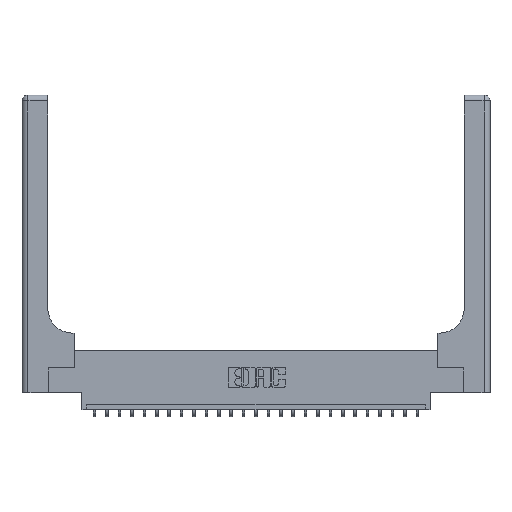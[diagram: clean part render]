
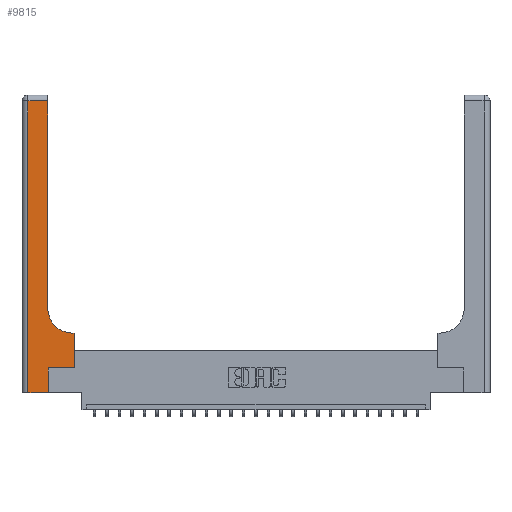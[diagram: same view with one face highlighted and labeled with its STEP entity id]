
A CAD part, top view. The second image highlights one B-rep face of the part: STEP entity #9815.
In plain terms, the highlighted planar face has unit normal (0, 0, 1).
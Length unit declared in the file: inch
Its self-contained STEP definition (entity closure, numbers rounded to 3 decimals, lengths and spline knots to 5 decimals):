
#491 = ORIENTED_EDGE ( 'NONE', *, *, #1760, .T. ) ;
#774 = PLANE ( 'NONE',  #8479 ) ;
#1011 = CIRCLE ( 'NONE', #23715, 0.25 ) ;
#1182 = LINE ( 'NONE', #22111, #23759 ) ;
#1273 = ORIENTED_EDGE ( 'NONE', *, *, #3967, .T. ) ;
#1760 = EDGE_CURVE ( 'NONE', #19154, #17649, #5342, .T. ) ;
#2073 = LINE ( 'NONE', #9685, #15956 ) ;
#2441 = DIRECTION ( 'NONE',  ( 1., 0., 0. ) ) ;
#2505 = CARTESIAN_POINT ( 'NONE',  ( 0.51, 0.85, 0.37 ) ) ;
#2872 = VERTEX_POINT ( 'NONE', #9540 ) ;
#3094 = EDGE_LOOP ( 'NONE', ( #10703, #1273, #18978, #21468, #18209, #21316, #21312, #491, #20974 ) ) ;
#3801 = CARTESIAN_POINT ( 'NONE',  ( 0.06, 2.94, 0.37 ) ) ;
#3824 = VERTEX_POINT ( 'NONE', #4258 ) ;
#3967 = EDGE_CURVE ( 'NONE', #21462, #16790, #12700, .T. ) ;
#4244 = CARTESIAN_POINT ( 'NONE',  ( 0.06, 0., 0.37 ) ) ;
#4258 = CARTESIAN_POINT ( 'NONE',  ( 0.26, 0.85, 0.37 ) ) ;
#5223 = CARTESIAN_POINT ( 'NONE',  ( 0.528, 0.25, 0.37 ) ) ;
#5342 = LINE ( 'NONE', #15129, #18626 ) ;
#5750 = VERTEX_POINT ( 'NONE', #5223 ) ;
#6818 = DIRECTION ( 'NONE',  ( 0., 1., 0. ) ) ;
#6942 = LINE ( 'NONE', #23510, #23726 ) ;
#8479 = AXIS2_PLACEMENT_3D ( 'NONE', #19824, #8750, #10242 ) ;
#8647 = EDGE_CURVE ( 'NONE', #17649, #3824, #1011, .T. ) ;
#8750 = DIRECTION ( 'NONE',  ( 0., 0., -1. ) ) ;
#9474 = CARTESIAN_POINT ( 'NONE',  ( 0.26, 2.94, 0.37 ) ) ;
#9540 = CARTESIAN_POINT ( 'NONE',  ( 0.265, 0., 0.37 ) ) ;
#9685 = CARTESIAN_POINT ( 'NONE',  ( 0., 0., 0.37 ) ) ;
#9815 = ADVANCED_FACE ( 'NONE', ( #21569 ), #774, .F. ) ;
#9930 = CARTESIAN_POINT ( 'NONE',  ( 0.528, 0.6, 0.37 ) ) ;
#10104 = VECTOR ( 'NONE', #24048, 39.37008 ) ;
#10111 = DIRECTION ( 'NONE',  ( 1., 0., 0. ) ) ;
#10190 = VECTOR ( 'NONE', #23112, 39.37008 ) ;
#10242 = DIRECTION ( 'NONE',  ( -1., 0., 0. ) ) ;
#10245 = VERTEX_POINT ( 'NONE', #17662 ) ;
#10475 = CARTESIAN_POINT ( 'NONE',  ( 0., 2.94, 0.37 ) ) ;
#10532 = DIRECTION ( 'NONE',  ( 1., 0., 0. ) ) ;
#10703 = ORIENTED_EDGE ( 'NONE', *, *, #14187, .T. ) ;
#11820 = LINE ( 'NONE', #21167, #16382 ) ;
#12235 = CARTESIAN_POINT ( 'NONE',  ( 0.51, 0.6, 0.37 ) ) ;
#12700 = LINE ( 'NONE', #10475, #10104 ) ;
#14187 = EDGE_CURVE ( 'NONE', #3824, #21462, #6942, .T. ) ;
#14262 = LINE ( 'NONE', #14742, #19322 ) ;
#14393 = EDGE_CURVE ( 'NONE', #5750, #19154, #22991, .T. ) ;
#14742 = CARTESIAN_POINT ( 'NONE',  ( 0.06, 3., 0.37 ) ) ;
#15129 = CARTESIAN_POINT ( 'NONE',  ( 0.26, 0.6, 0.37 ) ) ;
#15630 = EDGE_CURVE ( 'NONE', #16790, #20341, #14262, .T. ) ;
#15956 = VECTOR ( 'NONE', #2441, 39.37008 ) ;
#16382 = VECTOR ( 'NONE', #19300, 39.37008 ) ;
#16790 = VERTEX_POINT ( 'NONE', #3801 ) ;
#16891 = DIRECTION ( 'NONE',  ( -1., 0., 0. ) ) ;
#17111 = CARTESIAN_POINT ( 'NONE',  ( 0.528, 0.25, 0.37 ) ) ;
#17148 = EDGE_CURVE ( 'NONE', #10245, #5750, #1182, .T. ) ;
#17649 = VERTEX_POINT ( 'NONE', #12235 ) ;
#17662 = CARTESIAN_POINT ( 'NONE',  ( 0.265, 0.25, 0.37 ) ) ;
#17939 = DIRECTION ( 'NONE',  ( 0., 0., -1. ) ) ;
#18209 = ORIENTED_EDGE ( 'NONE', *, *, #23195, .T. ) ;
#18626 = VECTOR ( 'NONE', #16891, 39.37008 ) ;
#18978 = ORIENTED_EDGE ( 'NONE', *, *, #15630, .T. ) ;
#19154 = VERTEX_POINT ( 'NONE', #9930 ) ;
#19300 = DIRECTION ( 'NONE',  ( 0., 1., 0. ) ) ;
#19322 = VECTOR ( 'NONE', #19887, 39.37008 ) ;
#19824 = CARTESIAN_POINT ( 'NONE',  ( 0., 3., 0.37 ) ) ;
#19887 = DIRECTION ( 'NONE',  ( 0., -1., 0. ) ) ;
#20341 = VERTEX_POINT ( 'NONE', #4244 ) ;
#20974 = ORIENTED_EDGE ( 'NONE', *, *, #8647, .T. ) ;
#21167 = CARTESIAN_POINT ( 'NONE',  ( 0.265, 0., 0.37 ) ) ;
#21312 = ORIENTED_EDGE ( 'NONE', *, *, #14393, .T. ) ;
#21316 = ORIENTED_EDGE ( 'NONE', *, *, #17148, .T. ) ;
#21462 = VERTEX_POINT ( 'NONE', #9474 ) ;
#21468 = ORIENTED_EDGE ( 'NONE', *, *, #23647, .T. ) ;
#21569 = FACE_OUTER_BOUND ( 'NONE', #3094, .T. ) ;
#22111 = CARTESIAN_POINT ( 'NONE',  ( 0.265, 0.25, 0.37 ) ) ;
#22991 = LINE ( 'NONE', #17111, #10190 ) ;
#23112 = DIRECTION ( 'NONE',  ( 0., 1., 0. ) ) ;
#23195 = EDGE_CURVE ( 'NONE', #2872, #10245, #11820, .T. ) ;
#23510 = CARTESIAN_POINT ( 'NONE',  ( 0.26, 3., 0.37 ) ) ;
#23647 = EDGE_CURVE ( 'NONE', #20341, #2872, #2073, .T. ) ;
#23715 = AXIS2_PLACEMENT_3D ( 'NONE', #2505, #17939, #10111 ) ;
#23726 = VECTOR ( 'NONE', #6818, 39.37008 ) ;
#23759 = VECTOR ( 'NONE', #10532, 39.37008 ) ;
#24048 = DIRECTION ( 'NONE',  ( -1., 0., 0. ) ) ;
